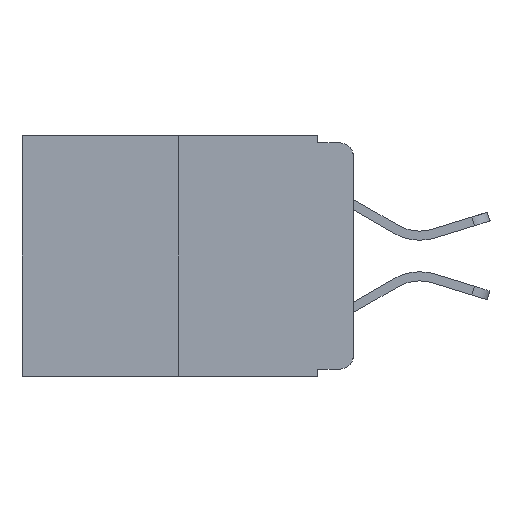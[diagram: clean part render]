
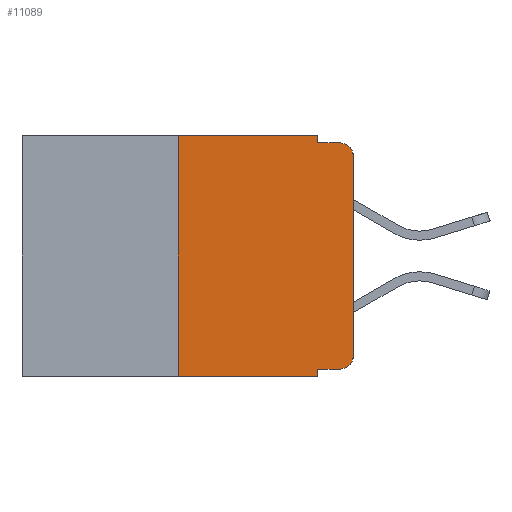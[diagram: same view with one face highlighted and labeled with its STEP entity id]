
A CAD part, left-side view. The second image highlights one B-rep face of the part: STEP entity #11089.
In plain terms, the highlighted planar face has unit normal (-1, 0, 0).
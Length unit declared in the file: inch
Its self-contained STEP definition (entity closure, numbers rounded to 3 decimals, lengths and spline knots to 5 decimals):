
#275 = VECTOR ( 'NONE', #913, 39.37008 ) ;
#454 = DIRECTION ( 'NONE',  ( 0., -1., 0. ) ) ;
#783 = EDGE_CURVE ( 'NONE', #8015, #11320, #25009, .T. ) ;
#913 = DIRECTION ( 'NONE',  ( 0., 0., 1. ) ) ;
#2857 = EDGE_CURVE ( 'NONE', #2905, #7051, #22368, .T. ) ;
#2905 = VERTEX_POINT ( 'NONE', #16773 ) ;
#3016 = EDGE_CURVE ( 'NONE', #6062, #2905, #19871, .T. ) ;
#3114 = CIRCLE ( 'NONE', #17173, 0.02 ) ;
#3320 = VECTOR ( 'NONE', #21033, 39.37008 ) ;
#3711 = CARTESIAN_POINT ( 'NONE',  ( 0., 0.051, -0.343 ) ) ;
#4136 = EDGE_CURVE ( 'NONE', #18820, #6062, #19504, .T. ) ;
#4235 = CARTESIAN_POINT ( 'NONE',  ( 0., 0.473, -0.343 ) ) ;
#4249 = LINE ( 'NONE', #18038, #24790 ) ;
#4448 = DIRECTION ( 'NONE',  ( -1., 0., 0. ) ) ;
#4491 = ORIENTED_EDGE ( 'NONE', *, *, #5850, .T. ) ;
#4582 = EDGE_CURVE ( 'NONE', #11320, #7051, #14846, .T. ) ;
#4729 = CARTESIAN_POINT ( 'NONE',  ( 0., 0.02, -0.333 ) ) ;
#4896 = ORIENTED_EDGE ( 'NONE', *, *, #19344, .T. ) ;
#5161 = CARTESIAN_POINT ( 'NONE',  ( 0., 0.473, 0. ) ) ;
#5269 = CARTESIAN_POINT ( 'NONE',  ( 0., 0.051, 0. ) ) ;
#5850 = EDGE_CURVE ( 'NONE', #6410, #25186, #21410, .T. ) ;
#6062 = VERTEX_POINT ( 'NONE', #5269 ) ;
#6385 = EDGE_CURVE ( 'NONE', #22372, #25186, #4249, .T. ) ;
#6410 = VERTEX_POINT ( 'NONE', #14242 ) ;
#7051 = VERTEX_POINT ( 'NONE', #20225 ) ;
#7173 = DIRECTION ( 'NONE',  ( 0., -1., 0. ) ) ;
#7263 = FACE_OUTER_BOUND ( 'NONE', #18032, .T. ) ;
#7738 = VECTOR ( 'NONE', #454, 39.37008 ) ;
#7935 = CARTESIAN_POINT ( 'NONE',  ( 0., 0.473, 0. ) ) ;
#8015 = VERTEX_POINT ( 'NONE', #22577 ) ;
#8887 = AXIS2_PLACEMENT_3D ( 'NONE', #16452, #4448, #18414 ) ;
#8895 = VECTOR ( 'NONE', #7173, 39.37008 ) ;
#9611 = CARTESIAN_POINT ( 'NONE',  ( 0., 0.02, -0.313 ) ) ;
#10906 = EDGE_CURVE ( 'NONE', #22372, #16562, #12963, .T. ) ;
#11089 = ADVANCED_FACE ( 'NONE', ( #7263 ), #19866, .F. ) ;
#11320 = VERTEX_POINT ( 'NONE', #16594 ) ;
#11634 = DIRECTION ( 'NONE',  ( 0., 0., -1. ) ) ;
#11992 = DIRECTION ( 'NONE',  ( 0., 0., -1. ) ) ;
#12963 = LINE ( 'NONE', #25152, #22230 ) ;
#13037 = ORIENTED_EDGE ( 'NONE', *, *, #783, .T. ) ;
#14242 = CARTESIAN_POINT ( 'NONE',  ( 0., 0.25, -0.343 ) ) ;
#14645 = ORIENTED_EDGE ( 'NONE', *, *, #15266, .F. ) ;
#14697 = CARTESIAN_POINT ( 'NONE',  ( 0., 0.051, -0.01 ) ) ;
#14716 = AXIS2_PLACEMENT_3D ( 'NONE', #7935, #23845, #11992 ) ;
#14846 = CIRCLE ( 'NONE', #8887, 0.02 ) ;
#15101 = CARTESIAN_POINT ( 'NONE',  ( 0., 0.051, 0. ) ) ;
#15266 = EDGE_CURVE ( 'NONE', #6410, #18820, #25647, .T. ) ;
#15423 = ORIENTED_EDGE ( 'NONE', *, *, #10906, .T. ) ;
#16191 = VECTOR ( 'NONE', #18293, 39.37008 ) ;
#16328 = ORIENTED_EDGE ( 'NONE', *, *, #3016, .F. ) ;
#16452 = CARTESIAN_POINT ( 'NONE',  ( 0., 0.02, -0.03 ) ) ;
#16562 = VERTEX_POINT ( 'NONE', #4729 ) ;
#16582 = ORIENTED_EDGE ( 'NONE', *, *, #4582, .T. ) ;
#16594 = CARTESIAN_POINT ( 'NONE',  ( 0., 0., -0.03 ) ) ;
#16773 = CARTESIAN_POINT ( 'NONE',  ( 0., 0.051, -0.01 ) ) ;
#17173 = AXIS2_PLACEMENT_3D ( 'NONE', #9611, #23503, #11634 ) ;
#17301 = DIRECTION ( 'NONE',  ( 0., -1., 0. ) ) ;
#18032 = EDGE_LOOP ( 'NONE', ( #13037, #16582, #18809, #16328, #21598, #14645, #4491, #19768, #15423, #4896 ) ) ;
#18038 = CARTESIAN_POINT ( 'NONE',  ( 0., 0.051, 0. ) ) ;
#18293 = DIRECTION ( 'NONE',  ( 0., -1., 0. ) ) ;
#18414 = DIRECTION ( 'NONE',  ( 0., 0., -1. ) ) ;
#18557 = CARTESIAN_POINT ( 'NONE',  ( 0., 0.051, -0.333 ) ) ;
#18809 = ORIENTED_EDGE ( 'NONE', *, *, #2857, .F. ) ;
#18820 = VERTEX_POINT ( 'NONE', #22077 ) ;
#18922 = CARTESIAN_POINT ( 'NONE',  ( 0., 0.25, 0. ) ) ;
#19025 = CARTESIAN_POINT ( 'NONE',  ( 0., 0., 0. ) ) ;
#19344 = EDGE_CURVE ( 'NONE', #16562, #8015, #3114, .T. ) ;
#19504 = LINE ( 'NONE', #5161, #8895 ) ;
#19750 = VECTOR ( 'NONE', #20594, 39.37008 ) ;
#19768 = ORIENTED_EDGE ( 'NONE', *, *, #6385, .F. ) ;
#19866 = PLANE ( 'NONE',  #14716 ) ;
#19871 = LINE ( 'NONE', #15101, #3320 ) ;
#20083 = DIRECTION ( 'NONE',  ( 0., 0., -1. ) ) ;
#20225 = CARTESIAN_POINT ( 'NONE',  ( 0., 0.02, -0.01 ) ) ;
#20594 = DIRECTION ( 'NONE',  ( 0., 0., 1. ) ) ;
#21033 = DIRECTION ( 'NONE',  ( 0., 0., -1. ) ) ;
#21410 = LINE ( 'NONE', #4235, #16191 ) ;
#21598 = ORIENTED_EDGE ( 'NONE', *, *, #4136, .F. ) ;
#22077 = CARTESIAN_POINT ( 'NONE',  ( 0., 0.25, 0. ) ) ;
#22230 = VECTOR ( 'NONE', #17301, 39.37008 ) ;
#22368 = LINE ( 'NONE', #14697, #7738 ) ;
#22372 = VERTEX_POINT ( 'NONE', #18557 ) ;
#22577 = CARTESIAN_POINT ( 'NONE',  ( 0., 0., -0.313 ) ) ;
#23503 = DIRECTION ( 'NONE',  ( -1., 0., 0. ) ) ;
#23845 = DIRECTION ( 'NONE',  ( 1., 0., 0. ) ) ;
#24790 = VECTOR ( 'NONE', #20083, 39.37008 ) ;
#25009 = LINE ( 'NONE', #19025, #19750 ) ;
#25152 = CARTESIAN_POINT ( 'NONE',  ( 0., 0.051, -0.333 ) ) ;
#25186 = VERTEX_POINT ( 'NONE', #3711 ) ;
#25647 = LINE ( 'NONE', #18922, #275 ) ;
